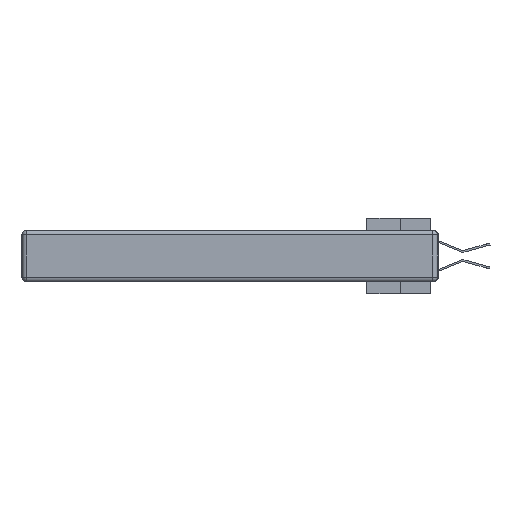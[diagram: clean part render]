
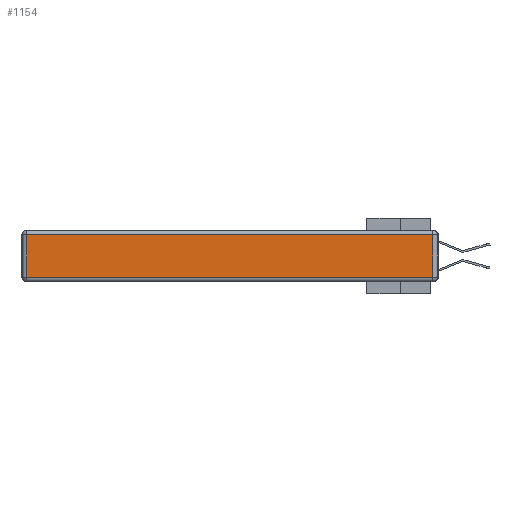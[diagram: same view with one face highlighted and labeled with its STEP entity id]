
A CAD part, left-side view. The second image highlights one B-rep face of the part: STEP entity #1154.
In plain terms, the highlighted planar face has unit normal (-1, 0, 0).
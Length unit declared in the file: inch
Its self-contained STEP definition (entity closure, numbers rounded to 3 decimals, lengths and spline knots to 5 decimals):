
#222 = DIRECTION ( 'NONE',  ( 0., 0., 1. ) ) ;
#598 = VECTOR ( 'NONE', #12489, 39.37008 ) ;
#743 = CARTESIAN_POINT ( 'NONE',  ( 0., 0., -0.313 ) ) ;
#1154 = ADVANCED_FACE ( 'NONE', ( #4465 ), #27512, .T. ) ;
#2887 = VERTEX_POINT ( 'NONE', #4510 ) ;
#3346 = ORIENTED_EDGE ( 'NONE', *, *, #5327, .T. ) ;
#3819 = LINE ( 'NONE', #11165, #22028 ) ;
#4465 = FACE_OUTER_BOUND ( 'NONE', #37403, .T. ) ;
#4510 = CARTESIAN_POINT ( 'NONE',  ( 0., 0.03, -0.313 ) ) ;
#5327 = EDGE_CURVE ( 'NONE', #2887, #30895, #11543, .T. ) ;
#5348 = CARTESIAN_POINT ( 'NONE',  ( 0., 2.75, -0.03 ) ) ;
#5580 = VERTEX_POINT ( 'NONE', #14155 ) ;
#8528 = LINE ( 'NONE', #743, #598 ) ;
#9443 = CARTESIAN_POINT ( 'NONE',  ( 0., 0.03, -0.03 ) ) ;
#11165 = CARTESIAN_POINT ( 'NONE',  ( 0., 2.72, -0.343 ) ) ;
#11543 = LINE ( 'NONE', #15268, #31189 ) ;
#11608 = ORIENTED_EDGE ( 'NONE', *, *, #24645, .T. ) ;
#12489 = DIRECTION ( 'NONE',  ( 0., -1., 0. ) ) ;
#13379 = VERTEX_POINT ( 'NONE', #20258 ) ;
#14155 = CARTESIAN_POINT ( 'NONE',  ( 0., 2.72, -0.313 ) ) ;
#14401 = DIRECTION ( 'NONE',  ( 0., 0., -1. ) ) ;
#14987 = CARTESIAN_POINT ( 'NONE',  ( 0., 0., -0.343 ) ) ;
#15268 = CARTESIAN_POINT ( 'NONE',  ( 0., 0.03, -0.343 ) ) ;
#15759 = LINE ( 'NONE', #5348, #30690 ) ;
#17069 = EDGE_CURVE ( 'NONE', #30895, #13379, #15759, .T. ) ;
#17234 = DIRECTION ( 'NONE',  ( 0., 1., 0. ) ) ;
#20258 = CARTESIAN_POINT ( 'NONE',  ( 0., 2.72, -0.03 ) ) ;
#21651 = ORIENTED_EDGE ( 'NONE', *, *, #17069, .T. ) ;
#22028 = VECTOR ( 'NONE', #14401, 39.37008 ) ;
#24645 = EDGE_CURVE ( 'NONE', #5580, #2887, #8528, .T. ) ;
#27512 = PLANE ( 'NONE',  #33811 ) ;
#28532 = ORIENTED_EDGE ( 'NONE', *, *, #33060, .T. ) ;
#30690 = VECTOR ( 'NONE', #17234, 39.37008 ) ;
#30895 = VERTEX_POINT ( 'NONE', #9443 ) ;
#31189 = VECTOR ( 'NONE', #36146, 39.37008 ) ;
#33060 = EDGE_CURVE ( 'NONE', #13379, #5580, #3819, .T. ) ;
#33811 = AXIS2_PLACEMENT_3D ( 'NONE', #14987, #35885, #222 ) ;
#35885 = DIRECTION ( 'NONE',  ( -1., 0., 0. ) ) ;
#36146 = DIRECTION ( 'NONE',  ( 0., 0., 1. ) ) ;
#37403 = EDGE_LOOP ( 'NONE', ( #11608, #3346, #21651, #28532 ) ) ;
